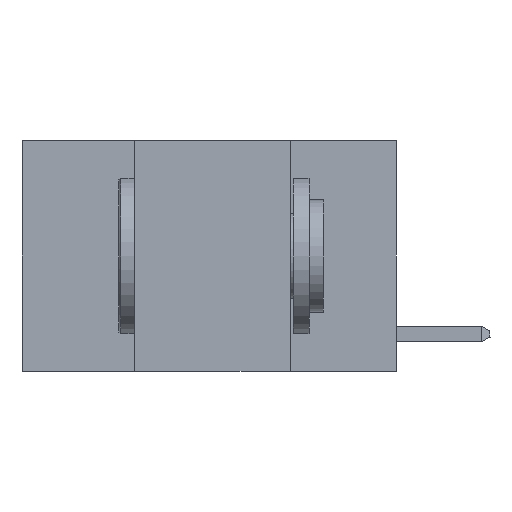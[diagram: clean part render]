
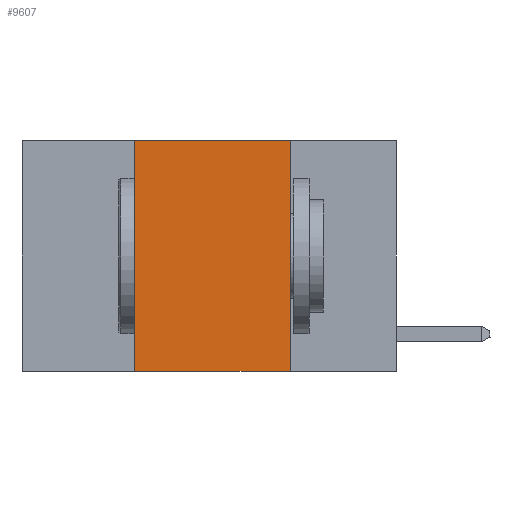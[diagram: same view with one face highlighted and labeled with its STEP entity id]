
A CAD part, left-side view. The second image highlights one B-rep face of the part: STEP entity #9607.
In plain terms, the highlighted planar face has unit normal (-1, 0, 0).
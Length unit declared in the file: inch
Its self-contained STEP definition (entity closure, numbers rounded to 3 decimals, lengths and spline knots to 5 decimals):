
#1358 = LINE ( 'NONE', #11912, #7238 ) ;
#1603 = FACE_OUTER_BOUND ( 'NONE', #4865, .T. ) ;
#3839 = DIRECTION ( 'NONE',  ( 0., 0., -1. ) ) ;
#4616 = DIRECTION ( 'NONE',  ( 0., -1., 0. ) ) ;
#4865 = EDGE_LOOP ( 'NONE', ( #13984, #26678, #9082, #10393 ) ) ;
#5210 = EDGE_CURVE ( 'NONE', #22612, #6531, #8893, .T. ) ;
#5955 = PLANE ( 'NONE',  #20470 ) ;
#6531 = VERTEX_POINT ( 'NONE', #22429 ) ;
#7238 = VECTOR ( 'NONE', #20504, 39.37008 ) ;
#8362 = LINE ( 'NONE', #19204, #13074 ) ;
#8893 = LINE ( 'NONE', #14809, #10442 ) ;
#9082 = ORIENTED_EDGE ( 'NONE', *, *, #21495, .F. ) ;
#9437 = CARTESIAN_POINT ( 'NONE',  ( 0., 0.6, -0.37 ) ) ;
#9607 = ADVANCED_FACE ( 'NONE', ( #1603 ), #5955, .F. ) ;
#10393 = ORIENTED_EDGE ( 'NONE', *, *, #20834, .T. ) ;
#10442 = VECTOR ( 'NONE', #12697, 39.37008 ) ;
#11912 = CARTESIAN_POINT ( 'NONE',  ( 0., 0.42, 0. ) ) ;
#12697 = DIRECTION ( 'NONE',  ( 0., -1., 0. ) ) ;
#13074 = VECTOR ( 'NONE', #19064, 39.37008 ) ;
#13984 = ORIENTED_EDGE ( 'NONE', *, *, #21551, .F. ) ;
#14552 = CARTESIAN_POINT ( 'NONE',  ( 0., 0.6, 0. ) ) ;
#14809 = CARTESIAN_POINT ( 'NONE',  ( 0., 0.6, 0. ) ) ;
#17874 = LINE ( 'NONE', #9437, #23006 ) ;
#19064 = DIRECTION ( 'NONE',  ( 0., 0., -1. ) ) ;
#19204 = CARTESIAN_POINT ( 'NONE',  ( 0., 0.17, 0. ) ) ;
#20470 = AXIS2_PLACEMENT_3D ( 'NONE', #14552, #23141, #3839 ) ;
#20504 = DIRECTION ( 'NONE',  ( 0., 0., 1. ) ) ;
#20834 = EDGE_CURVE ( 'NONE', #26549, #21406, #17874, .T. ) ;
#21406 = VERTEX_POINT ( 'NONE', #22490 ) ;
#21495 = EDGE_CURVE ( 'NONE', #26549, #22612, #1358, .T. ) ;
#21551 = EDGE_CURVE ( 'NONE', #6531, #21406, #8362, .T. ) ;
#22429 = CARTESIAN_POINT ( 'NONE',  ( 0., 0.17, 0. ) ) ;
#22490 = CARTESIAN_POINT ( 'NONE',  ( 0., 0.17, -0.37 ) ) ;
#22612 = VERTEX_POINT ( 'NONE', #24852 ) ;
#23006 = VECTOR ( 'NONE', #4616, 39.37008 ) ;
#23141 = DIRECTION ( 'NONE',  ( 1., 0., 0. ) ) ;
#23626 = CARTESIAN_POINT ( 'NONE',  ( 0., 0.42, -0.37 ) ) ;
#24852 = CARTESIAN_POINT ( 'NONE',  ( 0., 0.42, 0. ) ) ;
#26549 = VERTEX_POINT ( 'NONE', #23626 ) ;
#26678 = ORIENTED_EDGE ( 'NONE', *, *, #5210, .F. ) ;
